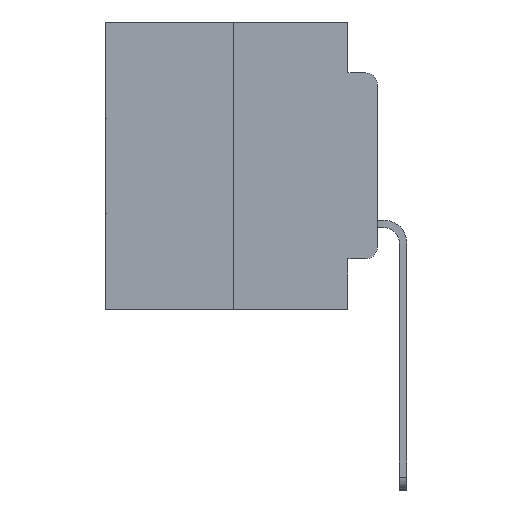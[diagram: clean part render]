
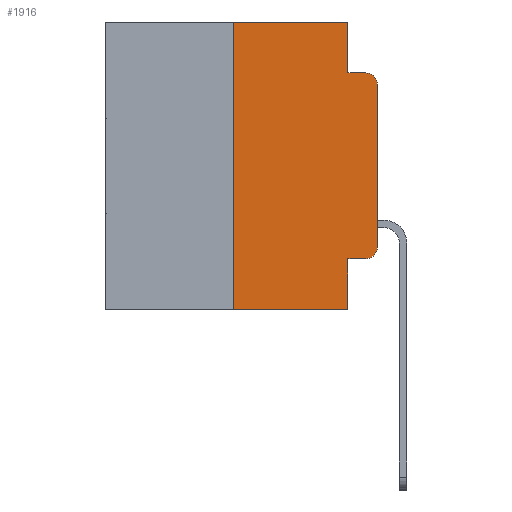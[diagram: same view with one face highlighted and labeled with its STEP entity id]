
A CAD part, left-side view. The second image highlights one B-rep face of the part: STEP entity #1916.
In plain terms, the highlighted planar face has unit normal (-1, 0, 0).
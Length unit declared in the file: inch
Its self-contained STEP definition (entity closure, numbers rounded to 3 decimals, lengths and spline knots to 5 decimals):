
#290 = DIRECTION ( 'NONE',  ( 0., 0., 1. ) ) ;
#334 = DIRECTION ( 'NONE',  ( 0., -1., 0. ) ) ;
#845 = EDGE_CURVE ( 'NONE', #22531, #26656, #3503, .T. ) ;
#1916 = ADVANCED_FACE ( 'NONE', ( #8431 ), #9921, .F. ) ;
#2054 = LINE ( 'NONE', #10928, #11962 ) ;
#2602 = DIRECTION ( 'NONE',  ( -1., 0., 0. ) ) ;
#2679 = ORIENTED_EDGE ( 'NONE', *, *, #11541, .T. ) ;
#3061 = ORIENTED_EDGE ( 'NONE', *, *, #27840, .F. ) ;
#3440 = DIRECTION ( 'NONE',  ( 1., 0., 0. ) ) ;
#3503 = LINE ( 'NONE', #16504, #25319 ) ;
#4596 = VERTEX_POINT ( 'NONE', #9319 ) ;
#5583 = EDGE_CURVE ( 'NONE', #10694, #4596, #2054, .T. ) ;
#6200 = LINE ( 'NONE', #13937, #17895 ) ;
#6546 = VERTEX_POINT ( 'NONE', #18615 ) ;
#6792 = LINE ( 'NONE', #17777, #23425 ) ;
#6880 = VECTOR ( 'NONE', #19949, 39.37008 ) ;
#7096 = EDGE_CURVE ( 'NONE', #4596, #10459, #25481, .T. ) ;
#7779 = VERTEX_POINT ( 'NONE', #8517 ) ;
#8431 = FACE_OUTER_BOUND ( 'NONE', #25479, .T. ) ;
#8517 = CARTESIAN_POINT ( 'NONE',  ( 0., 0.051, -0.5 ) ) ;
#9319 = CARTESIAN_POINT ( 'NONE',  ( 0., 0.051, -0.0885 ) ) ;
#9781 = DIRECTION ( 'NONE',  ( 0., -1., 0. ) ) ;
#9921 = PLANE ( 'NONE',  #20393 ) ;
#10092 = EDGE_CURVE ( 'NONE', #6546, #10459, #22097, .T. ) ;
#10147 = ORIENTED_EDGE ( 'NONE', *, *, #7096, .F. ) ;
#10459 = VERTEX_POINT ( 'NONE', #23587 ) ;
#10694 = VERTEX_POINT ( 'NONE', #26439 ) ;
#10928 = CARTESIAN_POINT ( 'NONE',  ( 0., 0.051, 0. ) ) ;
#11235 = DIRECTION ( 'NONE',  ( -1., 0., 0. ) ) ;
#11541 = EDGE_CURVE ( 'NONE', #21962, #6546, #21070, .T. ) ;
#11962 = VECTOR ( 'NONE', #19684, 39.37008 ) ;
#12344 = VERTEX_POINT ( 'NONE', #19176 ) ;
#12488 = CARTESIAN_POINT ( 'NONE',  ( 0., 0.25, -0.5 ) ) ;
#13742 = CARTESIAN_POINT ( 'NONE',  ( 0., 0.051, -0.0885 ) ) ;
#13937 = CARTESIAN_POINT ( 'NONE',  ( 0., 0.473, -0.5 ) ) ;
#13960 = DIRECTION ( 'NONE',  ( 0., 0., 1. ) ) ;
#14719 = CARTESIAN_POINT ( 'NONE',  ( 0., 0., -0.3915 ) ) ;
#15350 = VECTOR ( 'NONE', #290, 39.37008 ) ;
#15915 = DIRECTION ( 'NONE',  ( 0., -1., 0. ) ) ;
#15971 = CARTESIAN_POINT ( 'NONE',  ( 0., 0.02, -0.1085 ) ) ;
#16000 = DIRECTION ( 'NONE',  ( 0., 0., -1. ) ) ;
#16243 = CARTESIAN_POINT ( 'NONE',  ( 0., 0.25, 0. ) ) ;
#16504 = CARTESIAN_POINT ( 'NONE',  ( 0., 0.25, 0. ) ) ;
#17324 = ORIENTED_EDGE ( 'NONE', *, *, #20494, .F. ) ;
#17777 = CARTESIAN_POINT ( 'NONE',  ( 0., 0.051, 0. ) ) ;
#17778 = EDGE_CURVE ( 'NONE', #22531, #7779, #6200, .T. ) ;
#17895 = VECTOR ( 'NONE', #334, 39.37008 ) ;
#18007 = ORIENTED_EDGE ( 'NONE', *, *, #845, .F. ) ;
#18170 = DIRECTION ( 'NONE',  ( 0., 0., -1. ) ) ;
#18615 = CARTESIAN_POINT ( 'NONE',  ( 0., 0., -0.1085 ) ) ;
#19176 = CARTESIAN_POINT ( 'NONE',  ( 0., 0.051, -0.4115 ) ) ;
#19357 = ORIENTED_EDGE ( 'NONE', *, *, #17778, .T. ) ;
#19684 = DIRECTION ( 'NONE',  ( 0., 0., -1. ) ) ;
#19805 = VECTOR ( 'NONE', #9781, 39.37008 ) ;
#19933 = DIRECTION ( 'NONE',  ( 0., 0., -1. ) ) ;
#19949 = DIRECTION ( 'NONE',  ( 0., -1., 0. ) ) ;
#20328 = CARTESIAN_POINT ( 'NONE',  ( 0., 0., 0. ) ) ;
#20393 = AXIS2_PLACEMENT_3D ( 'NONE', #23015, #3440, #16000 ) ;
#20494 = EDGE_CURVE ( 'NONE', #26656, #10694, #26030, .T. ) ;
#20614 = CARTESIAN_POINT ( 'NONE',  ( 0., 0.473, 0. ) ) ;
#21070 = LINE ( 'NONE', #20328, #15350 ) ;
#21216 = AXIS2_PLACEMENT_3D ( 'NONE', #24094, #11235, #26228 ) ;
#21243 = CARTESIAN_POINT ( 'NONE',  ( 0., 0.02, -0.4115 ) ) ;
#21962 = VERTEX_POINT ( 'NONE', #14719 ) ;
#22006 = CARTESIAN_POINT ( 'NONE',  ( 0., 0.051, -0.4115 ) ) ;
#22097 = CIRCLE ( 'NONE', #22501, 0.02 ) ;
#22243 = EDGE_CURVE ( 'NONE', #26856, #21962, #22682, .T. ) ;
#22501 = AXIS2_PLACEMENT_3D ( 'NONE', #15971, #2602, #18170 ) ;
#22531 = VERTEX_POINT ( 'NONE', #12488 ) ;
#22682 = CIRCLE ( 'NONE', #21216, 0.02 ) ;
#23015 = CARTESIAN_POINT ( 'NONE',  ( 0., 0.473, 0. ) ) ;
#23425 = VECTOR ( 'NONE', #19933, 39.37008 ) ;
#23587 = CARTESIAN_POINT ( 'NONE',  ( 0., 0.02, -0.0885 ) ) ;
#24094 = CARTESIAN_POINT ( 'NONE',  ( 0., 0.02, -0.3915 ) ) ;
#24136 = LINE ( 'NONE', #22006, #6880 ) ;
#24831 = VECTOR ( 'NONE', #15915, 39.37008 ) ;
#25319 = VECTOR ( 'NONE', #13960, 39.37008 ) ;
#25479 = EDGE_LOOP ( 'NONE', ( #2679, #26594, #10147, #27896, #17324, #18007, #19357, #3061, #26943, #28231 ) ) ;
#25481 = LINE ( 'NONE', #13742, #24831 ) ;
#26030 = LINE ( 'NONE', #20614, #19805 ) ;
#26228 = DIRECTION ( 'NONE',  ( 0., 0., -1. ) ) ;
#26439 = CARTESIAN_POINT ( 'NONE',  ( 0., 0.051, 0. ) ) ;
#26440 = EDGE_CURVE ( 'NONE', #12344, #26856, #24136, .T. ) ;
#26594 = ORIENTED_EDGE ( 'NONE', *, *, #10092, .T. ) ;
#26656 = VERTEX_POINT ( 'NONE', #16243 ) ;
#26856 = VERTEX_POINT ( 'NONE', #21243 ) ;
#26943 = ORIENTED_EDGE ( 'NONE', *, *, #26440, .T. ) ;
#27840 = EDGE_CURVE ( 'NONE', #12344, #7779, #6792, .T. ) ;
#27896 = ORIENTED_EDGE ( 'NONE', *, *, #5583, .F. ) ;
#28231 = ORIENTED_EDGE ( 'NONE', *, *, #22243, .T. ) ;
